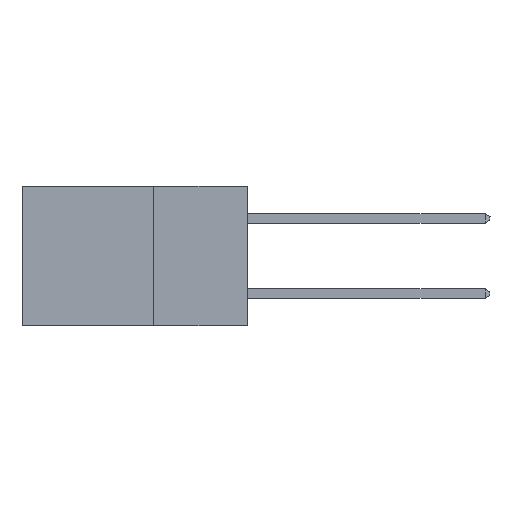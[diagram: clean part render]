
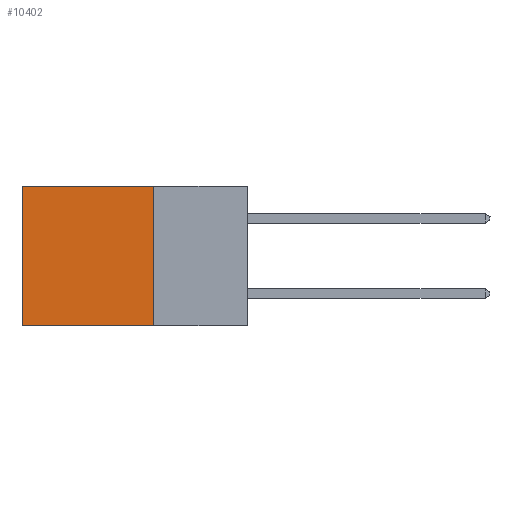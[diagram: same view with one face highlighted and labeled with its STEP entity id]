
A CAD part, left-side view. The second image highlights one B-rep face of the part: STEP entity #10402.
In plain terms, the highlighted planar face has unit normal (-1, 0, 0).
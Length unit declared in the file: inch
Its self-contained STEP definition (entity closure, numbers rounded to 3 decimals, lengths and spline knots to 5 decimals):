
#2185 = VECTOR ( 'NONE', #7535, 39.37008 ) ;
#2403 = CARTESIAN_POINT ( 'NONE',  ( 0.2615, 0.25, -0.37 ) ) ;
#2579 = EDGE_LOOP ( 'NONE', ( #3421, #27228, #16980, #26985 ) ) ;
#2699 = LINE ( 'NONE', #24284, #13776 ) ;
#2853 = VERTEX_POINT ( 'NONE', #13881 ) ;
#3421 = ORIENTED_EDGE ( 'NONE', *, *, #25768, .T. ) ;
#3726 = AXIS2_PLACEMENT_3D ( 'NONE', #25249, #14582, #19183 ) ;
#4059 = LINE ( 'NONE', #20868, #11458 ) ;
#5079 = DIRECTION ( 'NONE',  ( 0., 0., -1. ) ) ;
#5614 = CARTESIAN_POINT ( 'NONE',  ( 0.2615, 0.25, 0. ) ) ;
#6900 = CARTESIAN_POINT ( 'NONE',  ( 0.2615, 0.25, -0.37 ) ) ;
#7535 = DIRECTION ( 'NONE',  ( 0., 0., -1. ) ) ;
#10402 = ADVANCED_FACE ( 'NONE', ( #12767 ), #16675, .F. ) ;
#11220 = DIRECTION ( 'NONE',  ( 0., 1., 0. ) ) ;
#11458 = VECTOR ( 'NONE', #16790, 39.37008 ) ;
#11874 = VERTEX_POINT ( 'NONE', #6900 ) ;
#12767 = FACE_OUTER_BOUND ( 'NONE', #2579, .T. ) ;
#12805 = VECTOR ( 'NONE', #11220, 39.37008 ) ;
#13729 = EDGE_CURVE ( 'NONE', #11874, #14537, #21609, .T. ) ;
#13776 = VECTOR ( 'NONE', #5079, 39.37008 ) ;
#13881 = CARTESIAN_POINT ( 'NONE',  ( 0.2615, 0.6, 0. ) ) ;
#14009 = EDGE_CURVE ( 'NONE', #25757, #2853, #4059, .T. ) ;
#14537 = VERTEX_POINT ( 'NONE', #14642 ) ;
#14582 = DIRECTION ( 'NONE',  ( 1., 0., 0. ) ) ;
#14642 = CARTESIAN_POINT ( 'NONE',  ( 0.2615, 0.6, -0.37 ) ) ;
#16675 = PLANE ( 'NONE',  #3726 ) ;
#16790 = DIRECTION ( 'NONE',  ( 0., 1., 0. ) ) ;
#16980 = ORIENTED_EDGE ( 'NONE', *, *, #23672, .F. ) ;
#18190 = CARTESIAN_POINT ( 'NONE',  ( 0.2615, 0.6, -0.37 ) ) ;
#18734 = LINE ( 'NONE', #18190, #2185 ) ;
#19183 = DIRECTION ( 'NONE',  ( 0., 0., -1. ) ) ;
#20868 = CARTESIAN_POINT ( 'NONE',  ( 0.2615, 0.25, 0. ) ) ;
#21609 = LINE ( 'NONE', #2403, #12805 ) ;
#23672 = EDGE_CURVE ( 'NONE', #25757, #11874, #2699, .T. ) ;
#24284 = CARTESIAN_POINT ( 'NONE',  ( 0.2615, 0.25, -0.37 ) ) ;
#25249 = CARTESIAN_POINT ( 'NONE',  ( 0.2615, 0.25, -0.37 ) ) ;
#25757 = VERTEX_POINT ( 'NONE', #5614 ) ;
#25768 = EDGE_CURVE ( 'NONE', #2853, #14537, #18734, .T. ) ;
#26985 = ORIENTED_EDGE ( 'NONE', *, *, #14009, .T. ) ;
#27228 = ORIENTED_EDGE ( 'NONE', *, *, #13729, .F. ) ;
